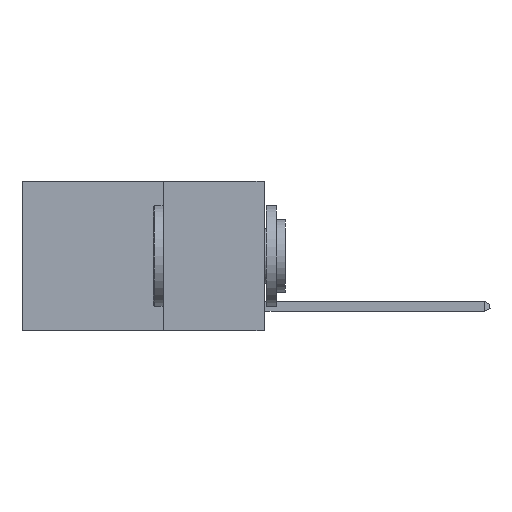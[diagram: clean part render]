
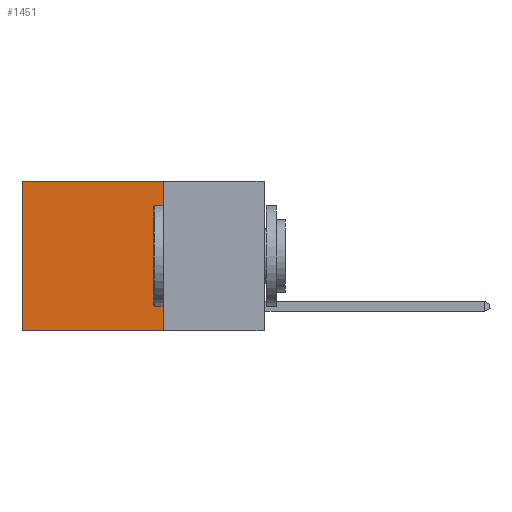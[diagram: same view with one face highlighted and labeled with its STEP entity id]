
A CAD part, left-side view. The second image highlights one B-rep face of the part: STEP entity #1451.
In plain terms, the highlighted planar face has unit normal (-1, 0, 0).
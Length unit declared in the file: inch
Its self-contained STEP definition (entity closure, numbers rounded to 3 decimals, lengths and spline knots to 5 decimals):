
#11 = CARTESIAN_POINT ( 'NONE',  ( 0.2625, 0.6, -0.37 ) ) ;
#100 = ORIENTED_EDGE ( 'NONE', *, *, #9007, .T. ) ;
#605 = VERTEX_POINT ( 'NONE', #11 ) ;
#804 = EDGE_CURVE ( 'NONE', #3722, #5320, #2261, .T. ) ;
#1415 = FACE_OUTER_BOUND ( 'NONE', #5957, .T. ) ;
#1451 = ADVANCED_FACE ( 'NONE', ( #1415 ), #7925, .F. ) ;
#1536 = VECTOR ( 'NONE', #6602, 39.37008 ) ;
#1683 = CARTESIAN_POINT ( 'NONE',  ( 0.2625, 0.6, 0. ) ) ;
#1862 = DIRECTION ( 'NONE',  ( 0., 1., 0. ) ) ;
#2076 = LINE ( 'NONE', #15260, #1536 ) ;
#2261 = LINE ( 'NONE', #13063, #5801 ) ;
#2752 = DIRECTION ( 'NONE',  ( 1., 0., 0. ) ) ;
#3722 = VERTEX_POINT ( 'NONE', #10812 ) ;
#5320 = VERTEX_POINT ( 'NONE', #6627 ) ;
#5801 = VECTOR ( 'NONE', #18231, 39.37008 ) ;
#5957 = EDGE_LOOP ( 'NONE', ( #100, #6145, #18933, #20767 ) ) ;
#6127 = EDGE_CURVE ( 'NONE', #3722, #14364, #18865, .T. ) ;
#6145 = ORIENTED_EDGE ( 'NONE', *, *, #11332, .F. ) ;
#6536 = VECTOR ( 'NONE', #22363, 39.37008 ) ;
#6602 = DIRECTION ( 'NONE',  ( 0., 1., 0. ) ) ;
#6627 = CARTESIAN_POINT ( 'NONE',  ( 0.2625, 0.25, -0.37 ) ) ;
#7090 = LINE ( 'NONE', #1683, #6536 ) ;
#7181 = AXIS2_PLACEMENT_3D ( 'NONE', #9692, #2752, #14906 ) ;
#7925 = PLANE ( 'NONE',  #7181 ) ;
#9007 = EDGE_CURVE ( 'NONE', #14364, #605, #7090, .T. ) ;
#9692 = CARTESIAN_POINT ( 'NONE',  ( 0.2625, 0.25, 0. ) ) ;
#10812 = CARTESIAN_POINT ( 'NONE',  ( 0.2625, 0.25, 0. ) ) ;
#11332 = EDGE_CURVE ( 'NONE', #5320, #605, #2076, .T. ) ;
#13063 = CARTESIAN_POINT ( 'NONE',  ( 0.2625, 0.25, 0. ) ) ;
#14364 = VERTEX_POINT ( 'NONE', #20369 ) ;
#14906 = DIRECTION ( 'NONE',  ( 0., 0., -1. ) ) ;
#15260 = CARTESIAN_POINT ( 'NONE',  ( 0.2625, 0.25, -0.37 ) ) ;
#15784 = CARTESIAN_POINT ( 'NONE',  ( 0.2625, 0.25, 0. ) ) ;
#17791 = VECTOR ( 'NONE', #1862, 39.37008 ) ;
#18231 = DIRECTION ( 'NONE',  ( 0., 0., -1. ) ) ;
#18865 = LINE ( 'NONE', #15784, #17791 ) ;
#18933 = ORIENTED_EDGE ( 'NONE', *, *, #804, .F. ) ;
#20369 = CARTESIAN_POINT ( 'NONE',  ( 0.2625, 0.6, 0. ) ) ;
#20767 = ORIENTED_EDGE ( 'NONE', *, *, #6127, .T. ) ;
#22363 = DIRECTION ( 'NONE',  ( 0., 0., -1. ) ) ;
